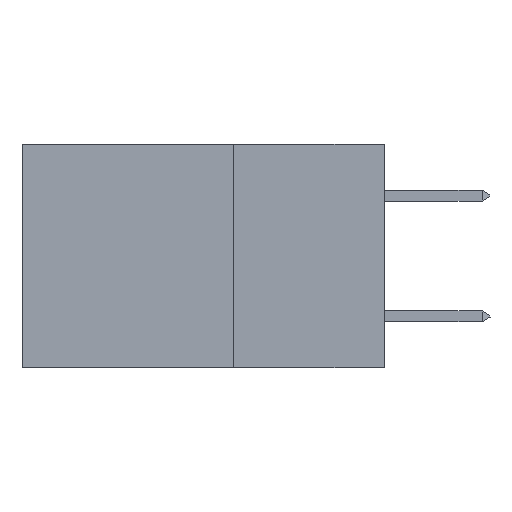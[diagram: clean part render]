
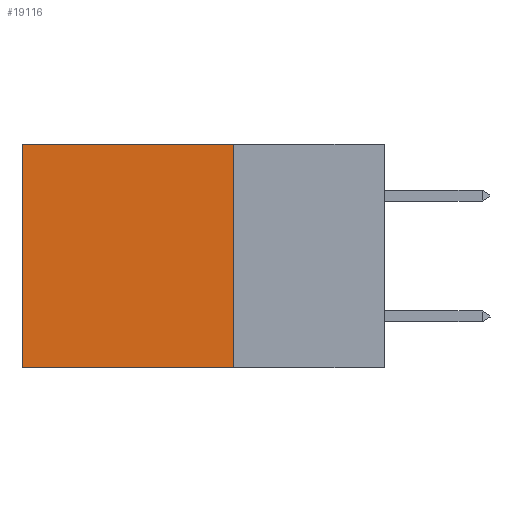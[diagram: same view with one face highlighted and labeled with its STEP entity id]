
A CAD part, left-side view. The second image highlights one B-rep face of the part: STEP entity #19116.
In plain terms, the highlighted planar face has unit normal (-1, 0, 0).
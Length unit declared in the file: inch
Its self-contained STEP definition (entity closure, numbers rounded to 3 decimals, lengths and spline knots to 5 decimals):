
#138 = VERTEX_POINT ( 'NONE', #13993 ) ;
#408 = DIRECTION ( 'NONE',  ( 0., 0., -1. ) ) ;
#681 = DIRECTION ( 'NONE',  ( 1., 0., 0. ) ) ;
#890 = CARTESIAN_POINT ( 'NONE',  ( 0.2875, 0.6, -0.37 ) ) ;
#1023 = LINE ( 'NONE', #11333, #16346 ) ;
#1146 = DIRECTION ( 'NONE',  ( 0., 0., -1. ) ) ;
#1385 = EDGE_CURVE ( 'NONE', #138, #15987, #15405, .T. ) ;
#2665 = DIRECTION ( 'NONE',  ( 0., 1., 0. ) ) ;
#3276 = ORIENTED_EDGE ( 'NONE', *, *, #6442, .T. ) ;
#5118 = EDGE_CURVE ( 'NONE', #16176, #10423, #1023, .T. ) ;
#5790 = CARTESIAN_POINT ( 'NONE',  ( 0.2875, 0.25, -0.37 ) ) ;
#5847 = VECTOR ( 'NONE', #22898, 39.37008 ) ;
#6442 = EDGE_CURVE ( 'NONE', #138, #16176, #13992, .T. ) ;
#7991 = CARTESIAN_POINT ( 'NONE',  ( 0.2875, 0.25, 0. ) ) ;
#8812 = ORIENTED_EDGE ( 'NONE', *, *, #18515, .F. ) ;
#9887 = PLANE ( 'NONE',  #14580 ) ;
#10423 = VERTEX_POINT ( 'NONE', #890 ) ;
#10537 = ORIENTED_EDGE ( 'NONE', *, *, #1385, .F. ) ;
#11294 = EDGE_LOOP ( 'NONE', ( #13368, #8812, #10537, #3276 ) ) ;
#11333 = CARTESIAN_POINT ( 'NONE',  ( 0.2875, 0.6, 0. ) ) ;
#12398 = CARTESIAN_POINT ( 'NONE',  ( 0.2875, 0.25, 0. ) ) ;
#13368 = ORIENTED_EDGE ( 'NONE', *, *, #5118, .T. ) ;
#13390 = CARTESIAN_POINT ( 'NONE',  ( 0.2875, 0.25, 0. ) ) ;
#13634 = DIRECTION ( 'NONE',  ( 0., 0., -1. ) ) ;
#13992 = LINE ( 'NONE', #7991, #5847 ) ;
#13993 = CARTESIAN_POINT ( 'NONE',  ( 0.2875, 0.25, 0. ) ) ;
#14154 = LINE ( 'NONE', #19359, #15326 ) ;
#14580 = AXIS2_PLACEMENT_3D ( 'NONE', #13390, #681, #13634 ) ;
#15326 = VECTOR ( 'NONE', #2665, 39.37008 ) ;
#15405 = LINE ( 'NONE', #12398, #17962 ) ;
#15987 = VERTEX_POINT ( 'NONE', #5790 ) ;
#16176 = VERTEX_POINT ( 'NONE', #20582 ) ;
#16346 = VECTOR ( 'NONE', #408, 39.37008 ) ;
#17574 = FACE_OUTER_BOUND ( 'NONE', #11294, .T. ) ;
#17962 = VECTOR ( 'NONE', #1146, 39.37008 ) ;
#18515 = EDGE_CURVE ( 'NONE', #15987, #10423, #14154, .T. ) ;
#19116 = ADVANCED_FACE ( 'NONE', ( #17574 ), #9887, .F. ) ;
#19359 = CARTESIAN_POINT ( 'NONE',  ( 0.2875, 0.25, -0.37 ) ) ;
#20582 = CARTESIAN_POINT ( 'NONE',  ( 0.2875, 0.6, 0. ) ) ;
#22898 = DIRECTION ( 'NONE',  ( 0., 1., 0. ) ) ;
